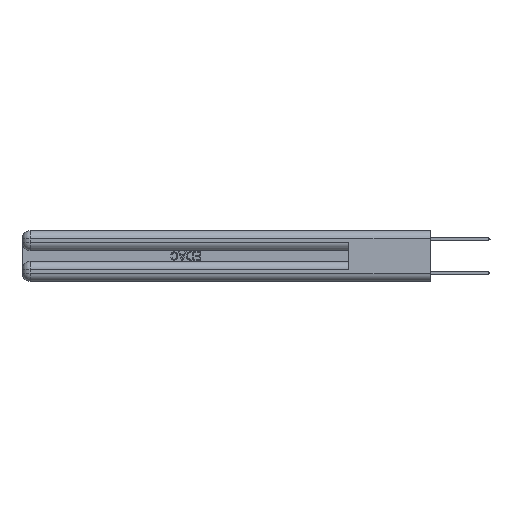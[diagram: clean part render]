
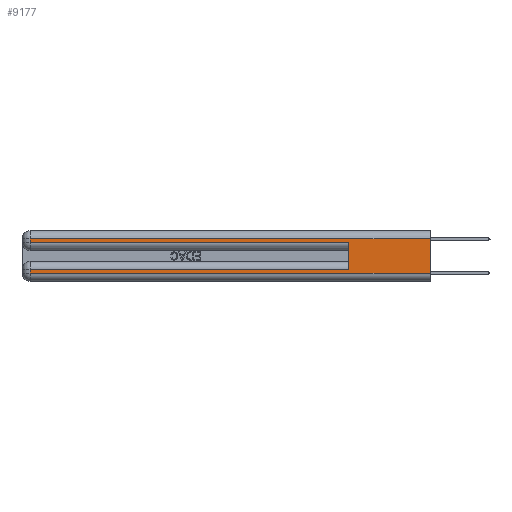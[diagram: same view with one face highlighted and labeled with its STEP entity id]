
A CAD part, left-side view. The second image highlights one B-rep face of the part: STEP entity #9177.
In plain terms, the highlighted planar face has unit normal (-1, 0, 0).
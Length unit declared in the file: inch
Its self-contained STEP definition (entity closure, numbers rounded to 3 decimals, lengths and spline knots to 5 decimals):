
#654 = LINE ( 'NONE', #6696, #7353 ) ;
#1038 = CARTESIAN_POINT ( 'NONE',  ( 0., 2.94, 0.37 ) ) ;
#1959 = DIRECTION ( 'NONE',  ( 0., 0., -1. ) ) ;
#2348 = ORIENTED_EDGE ( 'NONE', *, *, #7005, .T. ) ;
#2675 = LINE ( 'NONE', #29866, #22601 ) ;
#2862 = VERTEX_POINT ( 'NONE', #24213 ) ;
#3778 = EDGE_CURVE ( 'NONE', #12943, #2862, #36540, .T. ) ;
#5961 = CARTESIAN_POINT ( 'NONE',  ( 0., 0., 0.085 ) ) ;
#6142 = VECTOR ( 'NONE', #29424, 39.37008 ) ;
#6341 = CARTESIAN_POINT ( 'NONE',  ( 0., 0., 0.06 ) ) ;
#6470 = DIRECTION ( 'NONE',  ( 0., -1., 0. ) ) ;
#6550 = DIRECTION ( 'NONE',  ( 0., 0., -1. ) ) ;
#6696 = CARTESIAN_POINT ( 'NONE',  ( 0., 0.6, 0.145 ) ) ;
#7005 = EDGE_CURVE ( 'NONE', #2862, #16028, #13694, .T. ) ;
#7353 = VECTOR ( 'NONE', #21023, 39.37008 ) ;
#7817 = EDGE_CURVE ( 'NONE', #16028, #31038, #21366, .T. ) ;
#8203 = VECTOR ( 'NONE', #23253, 39.37008 ) ;
#8843 = CARTESIAN_POINT ( 'NONE',  ( 0., 0., 0.37 ) ) ;
#9177 = ADVANCED_FACE ( 'NONE', ( #26081 ), #28519, .F. ) ;
#9598 = CARTESIAN_POINT ( 'NONE',  ( 0., 2.94, 0.31 ) ) ;
#11596 = VECTOR ( 'NONE', #34150, 39.37008 ) ;
#11622 = ORIENTED_EDGE ( 'NONE', *, *, #7817, .T. ) ;
#12326 = EDGE_CURVE ( 'NONE', #12943, #25709, #654, .T. ) ;
#12943 = VERTEX_POINT ( 'NONE', #30317 ) ;
#13694 = LINE ( 'NONE', #1038, #6142 ) ;
#14374 = EDGE_CURVE ( 'NONE', #25765, #35927, #2675, .T. ) ;
#14974 = VECTOR ( 'NONE', #33262, 39.37008 ) ;
#15898 = AXIS2_PLACEMENT_3D ( 'NONE', #8843, #23838, #21006 ) ;
#16028 = VERTEX_POINT ( 'NONE', #30457 ) ;
#16389 = EDGE_CURVE ( 'NONE', #35927, #25709, #36767, .T. ) ;
#17246 = CARTESIAN_POINT ( 'NONE',  ( 0., 0., 0.31 ) ) ;
#17761 = VERTEX_POINT ( 'NONE', #34689 ) ;
#18065 = EDGE_CURVE ( 'NONE', #17761, #25765, #30387, .T. ) ;
#18961 = ORIENTED_EDGE ( 'NONE', *, *, #14374, .T. ) ;
#19749 = ORIENTED_EDGE ( 'NONE', *, *, #12326, .F. ) ;
#20017 = CARTESIAN_POINT ( 'NONE',  ( 0., 0., 0.06 ) ) ;
#20961 = CARTESIAN_POINT ( 'NONE',  ( 0., 2.94, 0.285 ) ) ;
#21006 = DIRECTION ( 'NONE',  ( 0., 0., -1. ) ) ;
#21023 = DIRECTION ( 'NONE',  ( 0., 0., 1. ) ) ;
#21366 = LINE ( 'NONE', #6341, #25764 ) ;
#22601 = VECTOR ( 'NONE', #1959, 39.37008 ) ;
#23222 = CARTESIAN_POINT ( 'NONE',  ( 0., 0., 0.37 ) ) ;
#23253 = DIRECTION ( 'NONE',  ( 0., 1., 0. ) ) ;
#23838 = DIRECTION ( 'NONE',  ( 1., 0., 0. ) ) ;
#24087 = ORIENTED_EDGE ( 'NONE', *, *, #16389, .T. ) ;
#24213 = CARTESIAN_POINT ( 'NONE',  ( 0., 2.94, 0.085 ) ) ;
#24225 = EDGE_CURVE ( 'NONE', #17761, #31038, #34026, .T. ) ;
#25709 = VERTEX_POINT ( 'NONE', #36512 ) ;
#25764 = VECTOR ( 'NONE', #6470, 39.37008 ) ;
#25765 = VERTEX_POINT ( 'NONE', #9598 ) ;
#26081 = FACE_OUTER_BOUND ( 'NONE', #31958, .T. ) ;
#28519 = PLANE ( 'NONE',  #15898 ) ;
#28625 = ORIENTED_EDGE ( 'NONE', *, *, #3778, .T. ) ;
#29424 = DIRECTION ( 'NONE',  ( 0., 0., -1. ) ) ;
#29866 = CARTESIAN_POINT ( 'NONE',  ( 0., 2.94, 0.37 ) ) ;
#30265 = CARTESIAN_POINT ( 'NONE',  ( 0., 0., 0.285 ) ) ;
#30317 = CARTESIAN_POINT ( 'NONE',  ( 0., 0.6, 0.085 ) ) ;
#30387 = LINE ( 'NONE', #17246, #8203 ) ;
#30457 = CARTESIAN_POINT ( 'NONE',  ( 0., 2.94, 0.06 ) ) ;
#31038 = VERTEX_POINT ( 'NONE', #20017 ) ;
#31768 = VECTOR ( 'NONE', #6550, 39.37008 ) ;
#31958 = EDGE_LOOP ( 'NONE', ( #32836, #35043, #18961, #24087, #19749, #28625, #2348, #11622 ) ) ;
#32836 = ORIENTED_EDGE ( 'NONE', *, *, #24225, .F. ) ;
#33262 = DIRECTION ( 'NONE',  ( 0., -1., 0. ) ) ;
#34026 = LINE ( 'NONE', #23222, #31768 ) ;
#34150 = DIRECTION ( 'NONE',  ( 0., 1., 0. ) ) ;
#34689 = CARTESIAN_POINT ( 'NONE',  ( 0., 0., 0.31 ) ) ;
#35043 = ORIENTED_EDGE ( 'NONE', *, *, #18065, .T. ) ;
#35927 = VERTEX_POINT ( 'NONE', #20961 ) ;
#36512 = CARTESIAN_POINT ( 'NONE',  ( 0., 0.6, 0.285 ) ) ;
#36540 = LINE ( 'NONE', #5961, #11596 ) ;
#36767 = LINE ( 'NONE', #30265, #14974 ) ;
